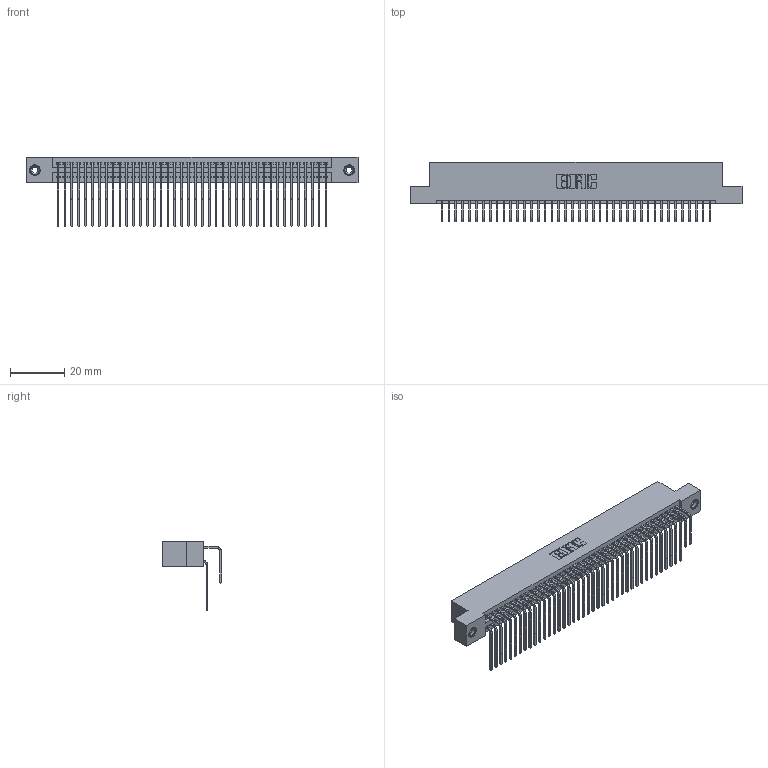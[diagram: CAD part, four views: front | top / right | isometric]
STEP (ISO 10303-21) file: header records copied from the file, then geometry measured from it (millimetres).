
FILE_DESCRIPTION (( 'STEP AP203' ), '1' );
FILE_NAME ('345-080-558-208.STEP', '2019-10-31T20:34:56', ( '' ), ( '' ), 'SwSTEP 2.0', 'SolidWorks 2016', '' );
FILE_SCHEMA (( 'CONFIG_CONTROL_DESIGN' ));
Length unit declared in the file: inch
Products named in the file (5): 345-292-001_558 559 Tail - 1; 345-250-001_345-250-003-102; 345-292-001_558 Tail - 2; 345 Part_Flush Mounting Lugs - 0.156 Dia-TI; 345-080-558-208
Assembly tree (83 placements, depth 2):
  345-080-558-208
    345 Part_Flush Mounting Lugs - 0.156 Dia-TI
    345-292-001_558 559 Tail - 1  x40
    345-292-001_558 Tail - 2  x40
    345-250-001_345-250-003-102  x2
Bounding box: 122.81 x 21.83 x 25.53 mm (x, y, z)
Volume: 12366.2 mm3; surface area: 20424.1 mm2
Topology: 83 solids, 83 shells, 4346 faces, 12877 edges, 8470 vertices
Faces by surface type: plane 2912, cylinder 1418, cone 12, torus 4
Entity records: 34492 total; most frequent: CARTESIAN_POINT 5810, ORIENTED_EDGE 5686, DIRECTION 5125, EDGE_CURVE 2843, LINE 2491, VECTOR 2491, VERTEX_POINT 1888, AXIS2_PLACEMENT_3D 1317
